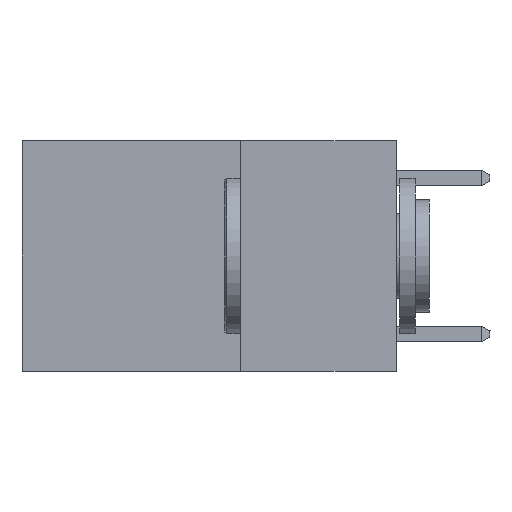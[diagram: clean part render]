
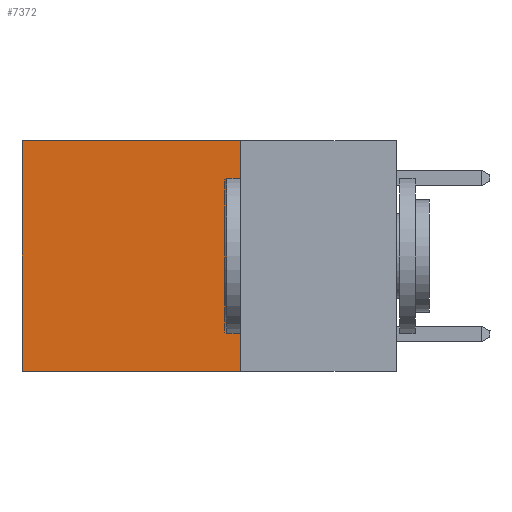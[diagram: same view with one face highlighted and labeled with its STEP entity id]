
A CAD part, left-side view. The second image highlights one B-rep face of the part: STEP entity #7372.
In plain terms, the highlighted planar face has unit normal (-1, 0, 0).
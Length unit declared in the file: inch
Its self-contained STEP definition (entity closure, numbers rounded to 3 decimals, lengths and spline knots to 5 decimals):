
#1929 = ORIENTED_EDGE ( 'NONE', *, *, #9150, .F. ) ;
#1982 = LINE ( 'NONE', #14300, #12350 ) ;
#3227 = DIRECTION ( 'NONE',  ( 0., 1., 0. ) ) ;
#3337 = CARTESIAN_POINT ( 'NONE',  ( 0.2625, 0.25, 0. ) ) ;
#3437 = CARTESIAN_POINT ( 'NONE',  ( 0.2625, 0.6, 0. ) ) ;
#3512 = CARTESIAN_POINT ( 'NONE',  ( 0.2625, 0.25, 0. ) ) ;
#3773 = VERTEX_POINT ( 'NONE', #6947 ) ;
#4085 = ORIENTED_EDGE ( 'NONE', *, *, #19017, .T. ) ;
#4110 = PLANE ( 'NONE',  #22596 ) ;
#5420 = DIRECTION ( 'NONE',  ( 0., 0., -1. ) ) ;
#6729 = EDGE_CURVE ( 'NONE', #14269, #20459, #1982, .T. ) ;
#6947 = CARTESIAN_POINT ( 'NONE',  ( 0.2625, 0.25, 0. ) ) ;
#7372 = ADVANCED_FACE ( 'NONE', ( #13287 ), #4110, .F. ) ;
#9150 = EDGE_CURVE ( 'NONE', #14958, #20459, #23133, .T. ) ;
#10387 = CARTESIAN_POINT ( 'NONE',  ( 0.2625, 0.25, 0. ) ) ;
#10799 = ORIENTED_EDGE ( 'NONE', *, *, #6729, .T. ) ;
#10956 = VECTOR ( 'NONE', #3227, 39.37008 ) ;
#11248 = EDGE_CURVE ( 'NONE', #3773, #14958, #16824, .T. ) ;
#11283 = VECTOR ( 'NONE', #5420, 39.37008 ) ;
#11517 = ORIENTED_EDGE ( 'NONE', *, *, #11248, .F. ) ;
#11948 = CARTESIAN_POINT ( 'NONE',  ( 0.2625, 0.6, -0.37 ) ) ;
#12350 = VECTOR ( 'NONE', #26399, 39.37008 ) ;
#12436 = DIRECTION ( 'NONE',  ( 0., 0., -1. ) ) ;
#13287 = FACE_OUTER_BOUND ( 'NONE', #15360, .T. ) ;
#13817 = DIRECTION ( 'NONE',  ( 0., 1., 0. ) ) ;
#14269 = VERTEX_POINT ( 'NONE', #3437 ) ;
#14300 = CARTESIAN_POINT ( 'NONE',  ( 0.2625, 0.6, 0. ) ) ;
#14958 = VERTEX_POINT ( 'NONE', #26144 ) ;
#15360 = EDGE_LOOP ( 'NONE', ( #10799, #1929, #11517, #4085 ) ) ;
#15649 = CARTESIAN_POINT ( 'NONE',  ( 0.2625, 0.25, -0.37 ) ) ;
#16824 = LINE ( 'NONE', #3337, #11283 ) ;
#19017 = EDGE_CURVE ( 'NONE', #3773, #14269, #21705, .T. ) ;
#20459 = VERTEX_POINT ( 'NONE', #11948 ) ;
#21705 = LINE ( 'NONE', #3512, #26343 ) ;
#22596 = AXIS2_PLACEMENT_3D ( 'NONE', #10387, #24669, #12436 ) ;
#23133 = LINE ( 'NONE', #15649, #10956 ) ;
#24669 = DIRECTION ( 'NONE',  ( 1., 0., 0. ) ) ;
#26144 = CARTESIAN_POINT ( 'NONE',  ( 0.2625, 0.25, -0.37 ) ) ;
#26343 = VECTOR ( 'NONE', #13817, 39.37008 ) ;
#26399 = DIRECTION ( 'NONE',  ( 0., 0., -1. ) ) ;
